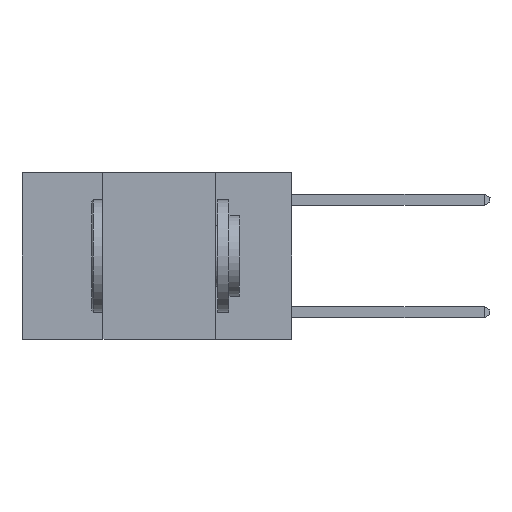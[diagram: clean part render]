
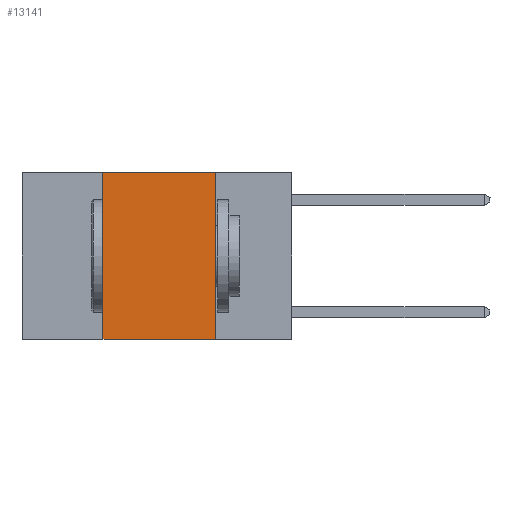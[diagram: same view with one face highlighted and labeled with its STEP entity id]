
A CAD part, left-side view. The second image highlights one B-rep face of the part: STEP entity #13141.
In plain terms, the highlighted planar face has unit normal (-1, 0, 0).
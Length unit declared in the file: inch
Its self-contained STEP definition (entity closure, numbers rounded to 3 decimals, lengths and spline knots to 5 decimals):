
#403 = CARTESIAN_POINT ( 'NONE',  ( 0., 0.6, -0.37 ) ) ;
#824 = ORIENTED_EDGE ( 'NONE', *, *, #23656, .T. ) ;
#1595 = CARTESIAN_POINT ( 'NONE',  ( 0., 0.6, 0. ) ) ;
#2329 = DIRECTION ( 'NONE',  ( 0., 0., -1. ) ) ;
#2834 = LINE ( 'NONE', #403, #9495 ) ;
#4017 = FACE_OUTER_BOUND ( 'NONE', #17517, .T. ) ;
#4433 = CARTESIAN_POINT ( 'NONE',  ( 0., 0.17, 0. ) ) ;
#6087 = DIRECTION ( 'NONE',  ( 0., -1., 0. ) ) ;
#6917 = VERTEX_POINT ( 'NONE', #24942 ) ;
#8077 = CARTESIAN_POINT ( 'NONE',  ( 0., 0.17, -0.37 ) ) ;
#8364 = EDGE_CURVE ( 'NONE', #19568, #6917, #25583, .T. ) ;
#9495 = VECTOR ( 'NONE', #14727, 39.37008 ) ;
#9789 = LINE ( 'NONE', #26854, #29624 ) ;
#11722 = AXIS2_PLACEMENT_3D ( 'NONE', #1595, #13826, #23662 ) ;
#12726 = ORIENTED_EDGE ( 'NONE', *, *, #8364, .F. ) ;
#13141 = ADVANCED_FACE ( 'NONE', ( #4017 ), #21244, .F. ) ;
#13826 = DIRECTION ( 'NONE',  ( 1., 0., 0. ) ) ;
#13930 = CARTESIAN_POINT ( 'NONE',  ( 0., 0.42, -0.37 ) ) ;
#14727 = DIRECTION ( 'NONE',  ( 0., -1., 0. ) ) ;
#16743 = VERTEX_POINT ( 'NONE', #13930 ) ;
#16831 = EDGE_CURVE ( 'NONE', #6917, #30895, #19566, .T. ) ;
#17316 = ORIENTED_EDGE ( 'NONE', *, *, #25074, .F. ) ;
#17517 = EDGE_LOOP ( 'NONE', ( #29371, #12726, #17316, #824 ) ) ;
#19276 = CARTESIAN_POINT ( 'NONE',  ( 0., 0.42, 0. ) ) ;
#19566 = LINE ( 'NONE', #4433, #23172 ) ;
#19568 = VERTEX_POINT ( 'NONE', #19276 ) ;
#21244 = PLANE ( 'NONE',  #11722 ) ;
#22045 = DIRECTION ( 'NONE',  ( 0., 0., 1. ) ) ;
#23172 = VECTOR ( 'NONE', #2329, 39.37008 ) ;
#23323 = CARTESIAN_POINT ( 'NONE',  ( 0., 0.6, 0. ) ) ;
#23403 = VECTOR ( 'NONE', #6087, 39.37008 ) ;
#23656 = EDGE_CURVE ( 'NONE', #16743, #30895, #2834, .T. ) ;
#23662 = DIRECTION ( 'NONE',  ( 0., 0., -1. ) ) ;
#24942 = CARTESIAN_POINT ( 'NONE',  ( 0., 0.17, 0. ) ) ;
#25074 = EDGE_CURVE ( 'NONE', #16743, #19568, #9789, .T. ) ;
#25583 = LINE ( 'NONE', #23323, #23403 ) ;
#26854 = CARTESIAN_POINT ( 'NONE',  ( 0., 0.42, 0. ) ) ;
#29371 = ORIENTED_EDGE ( 'NONE', *, *, #16831, .F. ) ;
#29624 = VECTOR ( 'NONE', #22045, 39.37008 ) ;
#30895 = VERTEX_POINT ( 'NONE', #8077 ) ;
